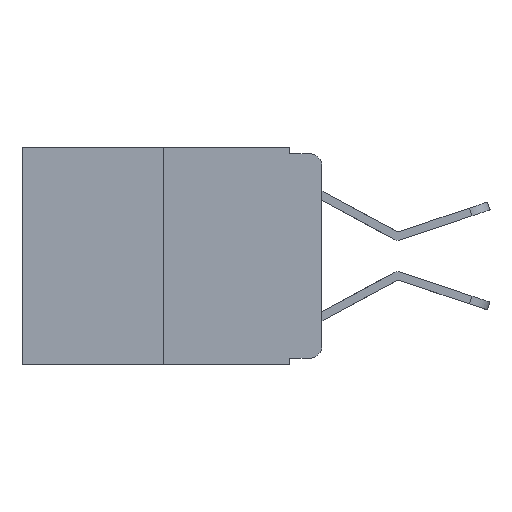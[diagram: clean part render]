
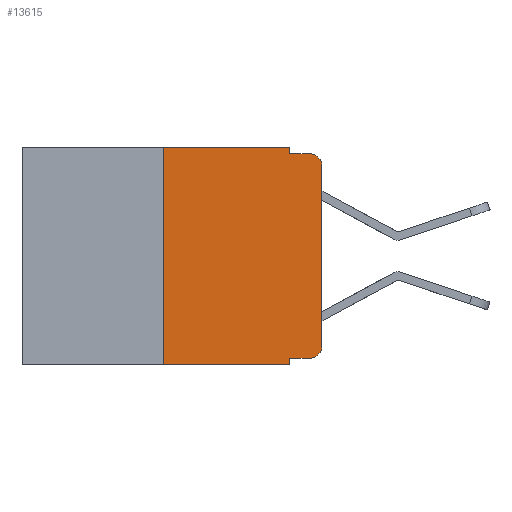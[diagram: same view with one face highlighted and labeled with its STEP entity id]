
A CAD part, left-side view. The second image highlights one B-rep face of the part: STEP entity #13615.
In plain terms, the highlighted planar face has unit normal (-1, 0, 0).
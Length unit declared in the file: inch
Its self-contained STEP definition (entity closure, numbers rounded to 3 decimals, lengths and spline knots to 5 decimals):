
#362 = CARTESIAN_POINT ( 'NONE',  ( 0., 0.473, 0. ) ) ;
#371 = DIRECTION ( 'NONE',  ( 0., 0., -1. ) ) ;
#697 = LINE ( 'NONE', #10151, #15734 ) ;
#914 = EDGE_CURVE ( 'NONE', #17378, #3424, #16002, .T. ) ;
#1373 = EDGE_CURVE ( 'NONE', #1674, #2436, #13623, .T. ) ;
#1674 = VERTEX_POINT ( 'NONE', #14014 ) ;
#2168 = CARTESIAN_POINT ( 'NONE',  ( 0., 0.473, 0. ) ) ;
#2173 = ORIENTED_EDGE ( 'NONE', *, *, #1373, .F. ) ;
#2191 = EDGE_CURVE ( 'NONE', #2436, #11586, #20389, .T. ) ;
#2215 = DIRECTION ( 'NONE',  ( -1., 0., 0. ) ) ;
#2432 = ORIENTED_EDGE ( 'NONE', *, *, #20696, .T. ) ;
#2436 = VERTEX_POINT ( 'NONE', #4977 ) ;
#2492 = CARTESIAN_POINT ( 'NONE',  ( 0., 0.02, -0.333 ) ) ;
#3424 = VERTEX_POINT ( 'NONE', #6176 ) ;
#3517 = VECTOR ( 'NONE', #4765, 39.37008 ) ;
#3659 = CARTESIAN_POINT ( 'NONE',  ( 0., 0.051, 0. ) ) ;
#3670 = EDGE_CURVE ( 'NONE', #11586, #17378, #12232, .T. ) ;
#4092 = ORIENTED_EDGE ( 'NONE', *, *, #13828, .T. ) ;
#4189 = DIRECTION ( 'NONE',  ( 0., 0., -1. ) ) ;
#4492 = ORIENTED_EDGE ( 'NONE', *, *, #20479, .T. ) ;
#4765 = DIRECTION ( 'NONE',  ( 0., -1., 0. ) ) ;
#4977 = CARTESIAN_POINT ( 'NONE',  ( 0., 0.25, 0. ) ) ;
#5740 = CARTESIAN_POINT ( 'NONE',  ( 0., 0., 0. ) ) ;
#5921 = ORIENTED_EDGE ( 'NONE', *, *, #2191, .F. ) ;
#6176 = CARTESIAN_POINT ( 'NONE',  ( 0., 0.02, -0.01 ) ) ;
#6602 = LINE ( 'NONE', #12830, #3517 ) ;
#6748 = CARTESIAN_POINT ( 'NONE',  ( 0., 0.051, 0. ) ) ;
#6840 = DIRECTION ( 'NONE',  ( 0., -1., 0. ) ) ;
#7377 = VECTOR ( 'NONE', #20520, 39.37008 ) ;
#7378 = CARTESIAN_POINT ( 'NONE',  ( 0., 0.02, -0.313 ) ) ;
#7426 = DIRECTION ( 'NONE',  ( 0., 0., 1. ) ) ;
#7472 = CARTESIAN_POINT ( 'NONE',  ( 0., 0., -0.03 ) ) ;
#8241 = VERTEX_POINT ( 'NONE', #2492 ) ;
#8285 = PLANE ( 'NONE',  #16017 ) ;
#8576 = DIRECTION ( 'NONE',  ( 0., 0., -1. ) ) ;
#8855 = VERTEX_POINT ( 'NONE', #13341 ) ;
#9042 = DIRECTION ( 'NONE',  ( -1., 0., 0. ) ) ;
#9143 = EDGE_CURVE ( 'NONE', #18496, #8241, #6602, .T. ) ;
#9492 = CARTESIAN_POINT ( 'NONE',  ( 0., 0.25, 0. ) ) ;
#9604 = ORIENTED_EDGE ( 'NONE', *, *, #9143, .T. ) ;
#9848 = CIRCLE ( 'NONE', #16814, 0.02 ) ;
#10151 = CARTESIAN_POINT ( 'NONE',  ( 0., 0.051, 0. ) ) ;
#10572 = CARTESIAN_POINT ( 'NONE',  ( 0., 0.473, -0.343 ) ) ;
#10900 = VECTOR ( 'NONE', #18542, 39.37008 ) ;
#10916 = CIRCLE ( 'NONE', #12025, 0.02 ) ;
#11502 = DIRECTION ( 'NONE',  ( 0., 0., 1. ) ) ;
#11586 = VERTEX_POINT ( 'NONE', #6748 ) ;
#11648 = DIRECTION ( 'NONE',  ( 1., 0., 0. ) ) ;
#12025 = AXIS2_PLACEMENT_3D ( 'NONE', #20433, #2215, #13790 ) ;
#12232 = LINE ( 'NONE', #3659, #10900 ) ;
#12830 = CARTESIAN_POINT ( 'NONE',  ( 0., 0.051, -0.333 ) ) ;
#13161 = CARTESIAN_POINT ( 'NONE',  ( 0., 0.051, -0.01 ) ) ;
#13341 = CARTESIAN_POINT ( 'NONE',  ( 0., 0., -0.313 ) ) ;
#13615 = ADVANCED_FACE ( 'NONE', ( #16481 ), #8285, .F. ) ;
#13623 = LINE ( 'NONE', #9492, #20680 ) ;
#13790 = DIRECTION ( 'NONE',  ( 0., 0., -1. ) ) ;
#13828 = EDGE_CURVE ( 'NONE', #1674, #16331, #20664, .T. ) ;
#13899 = LINE ( 'NONE', #5740, #20677 ) ;
#14014 = CARTESIAN_POINT ( 'NONE',  ( 0., 0.25, -0.343 ) ) ;
#14752 = CARTESIAN_POINT ( 'NONE',  ( 0., 0.051, -0.01 ) ) ;
#14759 = DIRECTION ( 'NONE',  ( 0., -1., 0. ) ) ;
#14966 = VECTOR ( 'NONE', #14759, 39.37008 ) ;
#15734 = VECTOR ( 'NONE', #371, 39.37008 ) ;
#16002 = LINE ( 'NONE', #13161, #14966 ) ;
#16017 = AXIS2_PLACEMENT_3D ( 'NONE', #362, #11648, #8576 ) ;
#16112 = ORIENTED_EDGE ( 'NONE', *, *, #3670, .F. ) ;
#16331 = VERTEX_POINT ( 'NONE', #17410 ) ;
#16481 = FACE_OUTER_BOUND ( 'NONE', #18187, .T. ) ;
#16567 = ORIENTED_EDGE ( 'NONE', *, *, #18597, .F. ) ;
#16814 = AXIS2_PLACEMENT_3D ( 'NONE', #7378, #9042, #4189 ) ;
#17378 = VERTEX_POINT ( 'NONE', #14752 ) ;
#17410 = CARTESIAN_POINT ( 'NONE',  ( 0., 0.051, -0.343 ) ) ;
#18187 = EDGE_LOOP ( 'NONE', ( #19910, #4492, #19122, #16112, #5921, #2173, #4092, #16567, #9604, #2432 ) ) ;
#18496 = VERTEX_POINT ( 'NONE', #19941 ) ;
#18542 = DIRECTION ( 'NONE',  ( 0., 0., -1. ) ) ;
#18597 = EDGE_CURVE ( 'NONE', #18496, #16331, #697, .T. ) ;
#18754 = EDGE_CURVE ( 'NONE', #8855, #20575, #13899, .T. ) ;
#18803 = VECTOR ( 'NONE', #6840, 39.37008 ) ;
#19122 = ORIENTED_EDGE ( 'NONE', *, *, #914, .F. ) ;
#19910 = ORIENTED_EDGE ( 'NONE', *, *, #18754, .T. ) ;
#19941 = CARTESIAN_POINT ( 'NONE',  ( 0., 0.051, -0.333 ) ) ;
#20389 = LINE ( 'NONE', #2168, #18803 ) ;
#20433 = CARTESIAN_POINT ( 'NONE',  ( 0., 0.02, -0.03 ) ) ;
#20479 = EDGE_CURVE ( 'NONE', #20575, #3424, #10916, .T. ) ;
#20520 = DIRECTION ( 'NONE',  ( 0., -1., 0. ) ) ;
#20575 = VERTEX_POINT ( 'NONE', #7472 ) ;
#20664 = LINE ( 'NONE', #10572, #7377 ) ;
#20677 = VECTOR ( 'NONE', #7426, 39.37008 ) ;
#20680 = VECTOR ( 'NONE', #11502, 39.37008 ) ;
#20696 = EDGE_CURVE ( 'NONE', #8241, #8855, #9848, .T. ) ;
